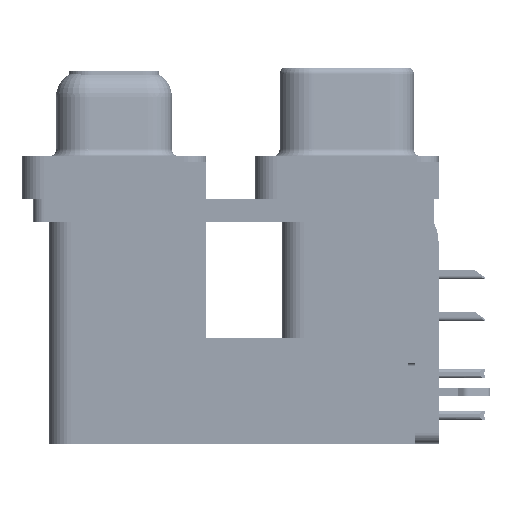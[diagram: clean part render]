
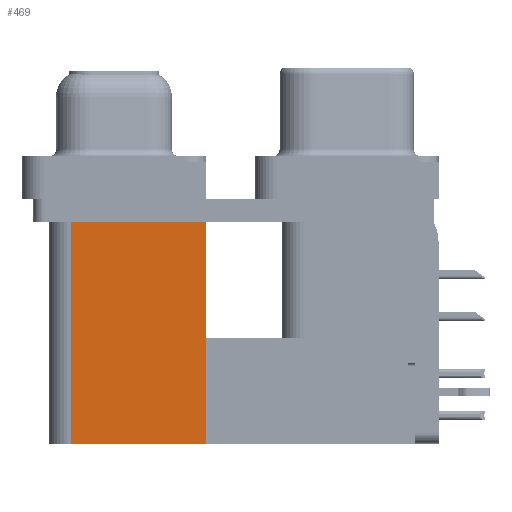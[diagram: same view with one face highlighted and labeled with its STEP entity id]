
A CAD part, left-side view. The second image highlights one B-rep face of the part: STEP entity #469.
In plain terms, the highlighted planar face has unit normal (-1, 0, 0).
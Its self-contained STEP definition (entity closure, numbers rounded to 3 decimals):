
#469 = ADVANCED_FACE ( 'NONE', ( #14638 ), #32151, .F. ) ;
#1407 = DIRECTION ( 'NONE',  ( 1., 0., 0. ) ) ;
#3119 = ORIENTED_EDGE ( 'NONE', *, *, #10134, .F. ) ;
#4808 = LINE ( 'NONE', #9135, #12339 ) ;
#7075 = VECTOR ( 'NONE', #40139, 1000. ) ;
#7855 = ORIENTED_EDGE ( 'NONE', *, *, #25658, .T. ) ;
#9135 = CARTESIAN_POINT ( 'NONE',  ( 3.7, 18.8, -19.2 ) ) ;
#10077 = CARTESIAN_POINT ( 'NONE',  ( 3.7, 9.6, -2.5 ) ) ;
#10134 = EDGE_CURVE ( 'NONE', #39821, #22715, #4808, .T. ) ;
#10378 = ORIENTED_EDGE ( 'NONE', *, *, #20026, .T. ) ;
#10978 = AXIS2_PLACEMENT_3D ( 'NONE', #31558, #1407, #14342 ) ;
#12339 = VECTOR ( 'NONE', #22330, 1000. ) ;
#13708 = DIRECTION ( 'NONE',  ( 0., 1., 0. ) ) ;
#14342 = DIRECTION ( 'NONE',  ( 0., 0., -1. ) ) ;
#14615 = CARTESIAN_POINT ( 'NONE',  ( 3.7, 9.6, -19.2 ) ) ;
#14638 = FACE_OUTER_BOUND ( 'NONE', #29066, .T. ) ;
#15971 = EDGE_CURVE ( 'NONE', #18487, #39821, #16626, .T. ) ;
#16626 = LINE ( 'NONE', #18320, #26060 ) ;
#18320 = CARTESIAN_POINT ( 'NONE',  ( 3.7, 9.6, -19.2 ) ) ;
#18487 = VERTEX_POINT ( 'NONE', #23272 ) ;
#20026 = EDGE_CURVE ( 'NONE', #18487, #35116, #49319, .T. ) ;
#22330 = DIRECTION ( 'NONE',  ( 0., 0., 1. ) ) ;
#22715 = VERTEX_POINT ( 'NONE', #47315 ) ;
#23272 = CARTESIAN_POINT ( 'NONE',  ( 3.7, 9.6, -19.2 ) ) ;
#25658 = EDGE_CURVE ( 'NONE', #35116, #22715, #27863, .T. ) ;
#26060 = VECTOR ( 'NONE', #13708, 1000. ) ;
#27021 = CARTESIAN_POINT ( 'NONE',  ( 3.7, 18.8, -19.2 ) ) ;
#27863 = LINE ( 'NONE', #10077, #37551 ) ;
#29066 = EDGE_LOOP ( 'NONE', ( #7855, #3119, #49767, #10378 ) ) ;
#31558 = CARTESIAN_POINT ( 'NONE',  ( 3.7, 9.6, -19.2 ) ) ;
#32151 = PLANE ( 'NONE',  #10978 ) ;
#35116 = VERTEX_POINT ( 'NONE', #38972 ) ;
#37551 = VECTOR ( 'NONE', #40756, 1000. ) ;
#38972 = CARTESIAN_POINT ( 'NONE',  ( 3.7, 9.6, -2.5 ) ) ;
#39821 = VERTEX_POINT ( 'NONE', #27021 ) ;
#40139 = DIRECTION ( 'NONE',  ( 0., 0., 1. ) ) ;
#40756 = DIRECTION ( 'NONE',  ( 0., 1., 0. ) ) ;
#47315 = CARTESIAN_POINT ( 'NONE',  ( 3.7, 18.8, -2.5 ) ) ;
#49319 = LINE ( 'NONE', #14615, #7075 ) ;
#49767 = ORIENTED_EDGE ( 'NONE', *, *, #15971, .F. ) ;
